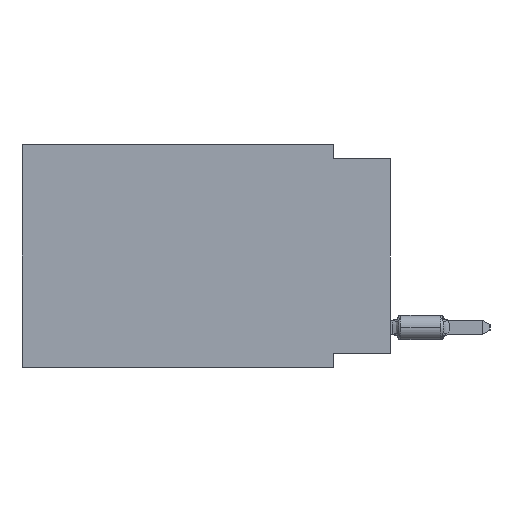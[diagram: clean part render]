
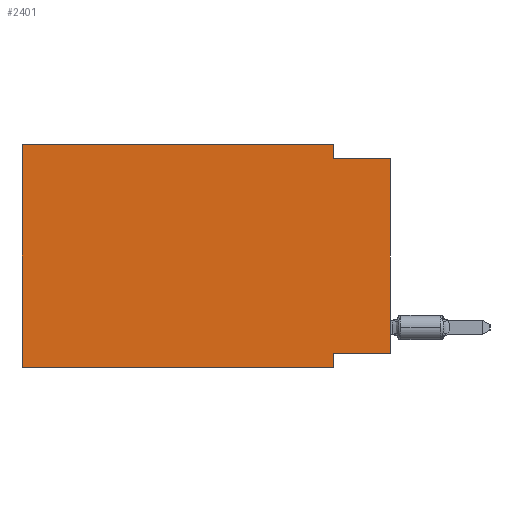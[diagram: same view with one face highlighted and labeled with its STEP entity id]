
A CAD part, left-side view. The second image highlights one B-rep face of the part: STEP entity #2401.
In plain terms, the highlighted planar face has unit normal (-1, 0, 0).
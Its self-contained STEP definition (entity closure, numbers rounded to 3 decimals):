
#2215 = VECTOR ( 'NONE', #9404, 1000. ) ;
#2253 = ORIENTED_EDGE ( 'NONE', *, *, #3620, .F. ) ;
#2401 = ADVANCED_FACE ( 'NONE', ( #31534 ), #24122, .F. ) ;
#2728 = CARTESIAN_POINT ( 'NONE',  ( 0., 2.54, -9.906 ) ) ;
#3222 = DIRECTION ( 'NONE',  ( 1., 0., 0. ) ) ;
#3552 = ORIENTED_EDGE ( 'NONE', *, *, #12799, .T. ) ;
#3620 = EDGE_CURVE ( 'NONE', #19892, #12044, #28023, .T. ) ;
#4835 = VERTEX_POINT ( 'NONE', #7409 ) ;
#4921 = DIRECTION ( 'NONE',  ( 0., 0., -1. ) ) ;
#5928 = DIRECTION ( 'NONE',  ( 0., 0., 1. ) ) ;
#6091 = CARTESIAN_POINT ( 'NONE',  ( 0., 16.383, 0. ) ) ;
#6712 = LINE ( 'NONE', #27618, #2215 ) ;
#7409 = CARTESIAN_POINT ( 'NONE',  ( 0., 16.383, -9.906 ) ) ;
#7721 = AXIS2_PLACEMENT_3D ( 'NONE', #6091, #3222, #21601 ) ;
#8558 = CARTESIAN_POINT ( 'NONE',  ( 0., 16.383, -9.906 ) ) ;
#8871 = LINE ( 'NONE', #26935, #25813 ) ;
#9404 = DIRECTION ( 'NONE',  ( 0., -1., 0. ) ) ;
#10914 = DIRECTION ( 'NONE',  ( 0., -1., 0. ) ) ;
#11296 = VERTEX_POINT ( 'NONE', #20488 ) ;
#11567 = ORIENTED_EDGE ( 'NONE', *, *, #30775, .F. ) ;
#12044 = VERTEX_POINT ( 'NONE', #31215 ) ;
#12205 = VECTOR ( 'NONE', #25491, 1000. ) ;
#12373 = CARTESIAN_POINT ( 'NONE',  ( 0., 2.54, 0. ) ) ;
#12799 = EDGE_CURVE ( 'NONE', #4835, #12044, #23569, .T. ) ;
#13537 = CARTESIAN_POINT ( 'NONE',  ( 0., 0., -0.635 ) ) ;
#13710 = VERTEX_POINT ( 'NONE', #13537 ) ;
#14051 = ORIENTED_EDGE ( 'NONE', *, *, #14796, .F. ) ;
#14796 = EDGE_CURVE ( 'NONE', #23585, #31484, #24302, .T. ) ;
#16010 = VECTOR ( 'NONE', #5928, 1000. ) ;
#16102 = LINE ( 'NONE', #19455, #20361 ) ;
#16658 = EDGE_CURVE ( 'NONE', #18822, #23585, #6712, .T. ) ;
#18822 = VERTEX_POINT ( 'NONE', #27736 ) ;
#19455 = CARTESIAN_POINT ( 'NONE',  ( 0., 0., -0.635 ) ) ;
#19549 = VECTOR ( 'NONE', #4921, 1000. ) ;
#19764 = CARTESIAN_POINT ( 'NONE',  ( 0., 2.54, -9.271 ) ) ;
#19892 = VERTEX_POINT ( 'NONE', #19764 ) ;
#20361 = VECTOR ( 'NONE', #29083, 1000. ) ;
#20488 = CARTESIAN_POINT ( 'NONE',  ( 0., 0., -9.271 ) ) ;
#21601 = DIRECTION ( 'NONE',  ( 0., 0., -1. ) ) ;
#21841 = ORIENTED_EDGE ( 'NONE', *, *, #31851, .T. ) ;
#21976 = ORIENTED_EDGE ( 'NONE', *, *, #16658, .F. ) ;
#22419 = DIRECTION ( 'NONE',  ( 0., 0., -1. ) ) ;
#22749 = ORIENTED_EDGE ( 'NONE', *, *, #30600, .F. ) ;
#22806 = CARTESIAN_POINT ( 'NONE',  ( 0., 0., -9.271 ) ) ;
#22896 = CARTESIAN_POINT ( 'NONE',  ( 0., 2.54, -0.635 ) ) ;
#23569 = LINE ( 'NONE', #8558, #32178 ) ;
#23585 = VERTEX_POINT ( 'NONE', #12373 ) ;
#23809 = CARTESIAN_POINT ( 'NONE',  ( 0., 16.383, 0. ) ) ;
#24122 = PLANE ( 'NONE',  #7721 ) ;
#24302 = LINE ( 'NONE', #32200, #32821 ) ;
#24434 = EDGE_CURVE ( 'NONE', #31484, #13710, #16102, .T. ) ;
#24581 = ORIENTED_EDGE ( 'NONE', *, *, #24434, .F. ) ;
#25017 = EDGE_LOOP ( 'NONE', ( #21841, #24581, #14051, #21976, #11567, #3552, #2253, #22749 ) ) ;
#25491 = DIRECTION ( 'NONE',  ( 0., 1., 0. ) ) ;
#25813 = VECTOR ( 'NONE', #31639, 1000. ) ;
#26935 = CARTESIAN_POINT ( 'NONE',  ( 0., 0., 0. ) ) ;
#27618 = CARTESIAN_POINT ( 'NONE',  ( 0., 16.383, 0. ) ) ;
#27736 = CARTESIAN_POINT ( 'NONE',  ( 0., 16.383, 0. ) ) ;
#28023 = LINE ( 'NONE', #2728, #19549 ) ;
#29083 = DIRECTION ( 'NONE',  ( 0., -1., 0. ) ) ;
#30193 = LINE ( 'NONE', #22806, #12205 ) ;
#30600 = EDGE_CURVE ( 'NONE', #11296, #19892, #30193, .T. ) ;
#30775 = EDGE_CURVE ( 'NONE', #4835, #18822, #31712, .T. ) ;
#31215 = CARTESIAN_POINT ( 'NONE',  ( 0., 2.54, -9.906 ) ) ;
#31484 = VERTEX_POINT ( 'NONE', #22896 ) ;
#31534 = FACE_OUTER_BOUND ( 'NONE', #25017, .T. ) ;
#31639 = DIRECTION ( 'NONE',  ( 0., 0., 1. ) ) ;
#31712 = LINE ( 'NONE', #23809, #16010 ) ;
#31851 = EDGE_CURVE ( 'NONE', #11296, #13710, #8871, .T. ) ;
#32178 = VECTOR ( 'NONE', #10914, 1000. ) ;
#32200 = CARTESIAN_POINT ( 'NONE',  ( 0., 2.54, 0. ) ) ;
#32821 = VECTOR ( 'NONE', #22419, 1000. ) ;
